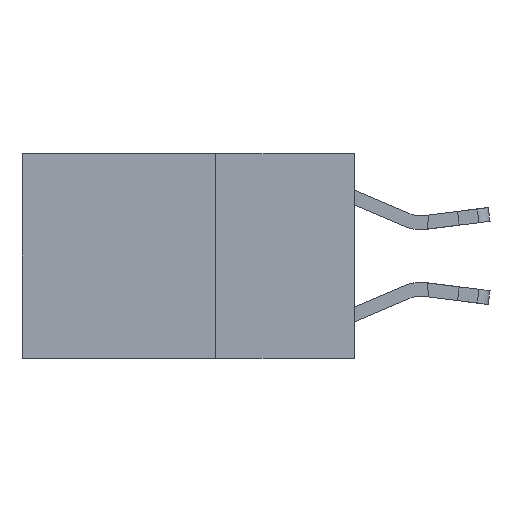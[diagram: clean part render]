
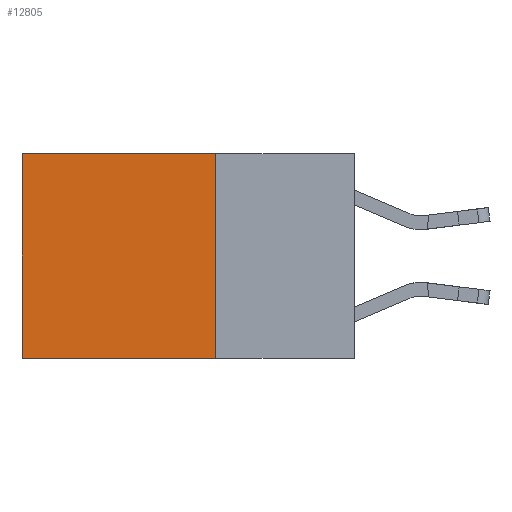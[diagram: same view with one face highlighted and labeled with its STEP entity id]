
A CAD part, left-side view. The second image highlights one B-rep face of the part: STEP entity #12805.
In plain terms, the highlighted planar face has unit normal (-1, 0, 0).
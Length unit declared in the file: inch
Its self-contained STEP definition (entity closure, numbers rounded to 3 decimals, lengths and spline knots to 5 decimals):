
#342 = VECTOR ( 'NONE', #6728, 39.37008 ) ;
#1104 = PLANE ( 'NONE',  #4070 ) ;
#1325 = CARTESIAN_POINT ( 'NONE',  ( 0.2625, 0.6, 0. ) ) ;
#1553 = DIRECTION ( 'NONE',  ( 0., 0., -1. ) ) ;
#2180 = CARTESIAN_POINT ( 'NONE',  ( 0.2625, 0.25, -0.37 ) ) ;
#2227 = LINE ( 'NONE', #10035, #3877 ) ;
#2720 = CARTESIAN_POINT ( 'NONE',  ( 0.2625, 0.25, 0. ) ) ;
#2886 = EDGE_CURVE ( 'NONE', #6906, #4048, #12453, .T. ) ;
#3682 = EDGE_CURVE ( 'NONE', #8251, #4048, #2227, .T. ) ;
#3729 = VECTOR ( 'NONE', #1553, 39.37008 ) ;
#3877 = VECTOR ( 'NONE', #12484, 39.37008 ) ;
#4048 = VERTEX_POINT ( 'NONE', #10791 ) ;
#4070 = AXIS2_PLACEMENT_3D ( 'NONE', #11428, #12461, #5557 ) ;
#5557 = DIRECTION ( 'NONE',  ( 0., 0., -1. ) ) ;
#5788 = EDGE_CURVE ( 'NONE', #9818, #6906, #13011, .T. ) ;
#6728 = DIRECTION ( 'NONE',  ( 0., 1., 0. ) ) ;
#6906 = VERTEX_POINT ( 'NONE', #7717 ) ;
#7232 = ORIENTED_EDGE ( 'NONE', *, *, #5788, .F. ) ;
#7717 = CARTESIAN_POINT ( 'NONE',  ( 0.2625, 0.25, -0.37 ) ) ;
#7749 = ORIENTED_EDGE ( 'NONE', *, *, #13738, .T. ) ;
#7878 = CARTESIAN_POINT ( 'NONE',  ( 0.2625, 0.25, 0. ) ) ;
#7887 = VECTOR ( 'NONE', #10204, 39.37008 ) ;
#8251 = VERTEX_POINT ( 'NONE', #1325 ) ;
#8972 = ORIENTED_EDGE ( 'NONE', *, *, #2886, .F. ) ;
#9818 = VERTEX_POINT ( 'NONE', #11131 ) ;
#10035 = CARTESIAN_POINT ( 'NONE',  ( 0.2625, 0.6, 0. ) ) ;
#10188 = ORIENTED_EDGE ( 'NONE', *, *, #3682, .T. ) ;
#10204 = DIRECTION ( 'NONE',  ( 0., 1., 0. ) ) ;
#10791 = CARTESIAN_POINT ( 'NONE',  ( 0.2625, 0.6, -0.37 ) ) ;
#11131 = CARTESIAN_POINT ( 'NONE',  ( 0.2625, 0.25, 0. ) ) ;
#11326 = LINE ( 'NONE', #7878, #7887 ) ;
#11428 = CARTESIAN_POINT ( 'NONE',  ( 0.2625, 0.25, 0. ) ) ;
#12045 = EDGE_LOOP ( 'NONE', ( #10188, #8972, #7232, #7749 ) ) ;
#12453 = LINE ( 'NONE', #2180, #342 ) ;
#12461 = DIRECTION ( 'NONE',  ( 1., 0., 0. ) ) ;
#12484 = DIRECTION ( 'NONE',  ( 0., 0., -1. ) ) ;
#12805 = ADVANCED_FACE ( 'NONE', ( #13593 ), #1104, .F. ) ;
#13011 = LINE ( 'NONE', #2720, #3729 ) ;
#13593 = FACE_OUTER_BOUND ( 'NONE', #12045, .T. ) ;
#13738 = EDGE_CURVE ( 'NONE', #9818, #8251, #11326, .T. ) ;
